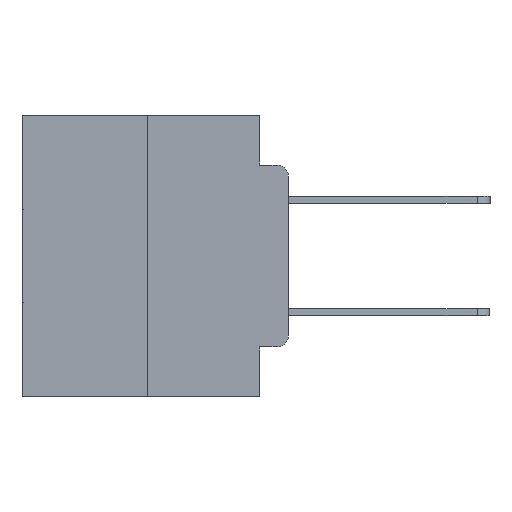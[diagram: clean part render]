
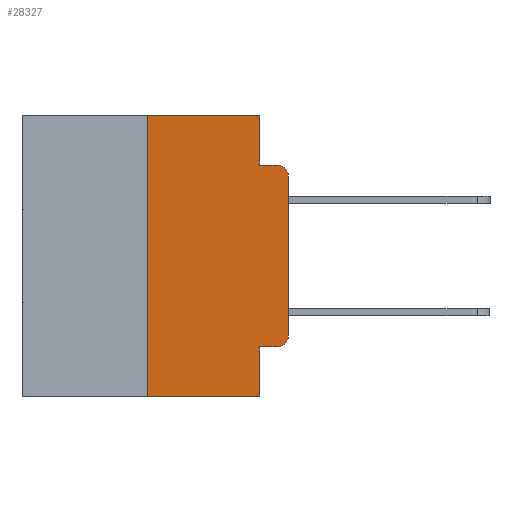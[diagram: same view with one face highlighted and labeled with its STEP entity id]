
A CAD part, left-side view. The second image highlights one B-rep face of the part: STEP entity #28327.
In plain terms, the highlighted planar face has unit normal (-1, 0, 0).
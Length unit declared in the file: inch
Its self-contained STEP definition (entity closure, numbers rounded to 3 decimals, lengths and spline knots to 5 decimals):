
#244 = CARTESIAN_POINT ( 'NONE',  ( 0., 0., -0.3915 ) ) ;
#656 = CARTESIAN_POINT ( 'NONE',  ( 0., 0.02, -0.1085 ) ) ;
#771 = DIRECTION ( 'NONE',  ( 0., 0., -1. ) ) ;
#1029 = ORIENTED_EDGE ( 'NONE', *, *, #26617, .F. ) ;
#1486 = CARTESIAN_POINT ( 'NONE',  ( 0., 0.25, 0. ) ) ;
#2059 = EDGE_CURVE ( 'NONE', #5785, #24473, #16417, .T. ) ;
#2586 = VERTEX_POINT ( 'NONE', #22466 ) ;
#2895 = CARTESIAN_POINT ( 'NONE',  ( 0., 0., 0. ) ) ;
#3025 = DIRECTION ( 'NONE',  ( 0., 0., -1. ) ) ;
#3027 = AXIS2_PLACEMENT_3D ( 'NONE', #18793, #18895, #5268 ) ;
#3279 = LINE ( 'NONE', #20834, #20783 ) ;
#3601 = VECTOR ( 'NONE', #771, 39.37008 ) ;
#3701 = CARTESIAN_POINT ( 'NONE',  ( 0., 0.02, -0.3915 ) ) ;
#3766 = LINE ( 'NONE', #16473, #15129 ) ;
#4317 = ORIENTED_EDGE ( 'NONE', *, *, #14441, .T. ) ;
#4804 = AXIS2_PLACEMENT_3D ( 'NONE', #656, #16676, #3025 ) ;
#5252 = DIRECTION ( 'NONE',  ( 0., -1., 0. ) ) ;
#5268 = DIRECTION ( 'NONE',  ( 0., 0., -1. ) ) ;
#5785 = VERTEX_POINT ( 'NONE', #28866 ) ;
#5810 = EDGE_LOOP ( 'NONE', ( #4317, #24004, #11480, #17840, #15767, #1029, #19303, #20393, #8933, #7186 ) ) ;
#5826 = VECTOR ( 'NONE', #21119, 39.37008 ) ;
#5998 = DIRECTION ( 'NONE',  ( 0., 0., -1. ) ) ;
#6046 = VERTEX_POINT ( 'NONE', #9480 ) ;
#7186 = ORIENTED_EDGE ( 'NONE', *, *, #18304, .T. ) ;
#7313 = CARTESIAN_POINT ( 'NONE',  ( 0., 0.051, -0.0885 ) ) ;
#7432 = VERTEX_POINT ( 'NONE', #16982 ) ;
#8602 = CIRCLE ( 'NONE', #4804, 0.02 ) ;
#8619 = CIRCLE ( 'NONE', #14096, 0.02 ) ;
#8933 = ORIENTED_EDGE ( 'NONE', *, *, #21608, .T. ) ;
#9033 = CARTESIAN_POINT ( 'NONE',  ( 0., 0.051, 0. ) ) ;
#9480 = CARTESIAN_POINT ( 'NONE',  ( 0., 0.051, -0.5 ) ) ;
#10533 = VECTOR ( 'NONE', #18191, 39.37008 ) ;
#10970 = VECTOR ( 'NONE', #14238, 39.37008 ) ;
#11480 = ORIENTED_EDGE ( 'NONE', *, *, #17508, .F. ) ;
#11672 = LINE ( 'NONE', #2895, #10970 ) ;
#11962 = EDGE_CURVE ( 'NONE', #13282, #23412, #8602, .T. ) ;
#11974 = CARTESIAN_POINT ( 'NONE',  ( 0., 0.473, -0.5 ) ) ;
#12280 = FACE_OUTER_BOUND ( 'NONE', #5810, .T. ) ;
#12442 = CARTESIAN_POINT ( 'NONE',  ( 0., 0.051, -0.0885 ) ) ;
#12578 = CARTESIAN_POINT ( 'NONE',  ( 0., 0.051, 0. ) ) ;
#13282 = VERTEX_POINT ( 'NONE', #19433 ) ;
#14096 = AXIS2_PLACEMENT_3D ( 'NONE', #3701, #19671, #5998 ) ;
#14238 = DIRECTION ( 'NONE',  ( 0., 0., 1. ) ) ;
#14441 = EDGE_CURVE ( 'NONE', #23753, #13282, #11672, .T. ) ;
#15129 = VECTOR ( 'NONE', #18777, 39.37008 ) ;
#15767 = ORIENTED_EDGE ( 'NONE', *, *, #16295, .F. ) ;
#16295 = EDGE_CURVE ( 'NONE', #25643, #5785, #3766, .T. ) ;
#16417 = LINE ( 'NONE', #12578, #3601 ) ;
#16473 = CARTESIAN_POINT ( 'NONE',  ( 0., 0.473, 0. ) ) ;
#16529 = LINE ( 'NONE', #1486, #22661 ) ;
#16585 = PLANE ( 'NONE',  #3027 ) ;
#16676 = DIRECTION ( 'NONE',  ( -1., 0., 0. ) ) ;
#16982 = CARTESIAN_POINT ( 'NONE',  ( 0., 0.051, -0.4115 ) ) ;
#17476 = DIRECTION ( 'NONE',  ( 0., 0., 1. ) ) ;
#17508 = EDGE_CURVE ( 'NONE', #24473, #23412, #25464, .T. ) ;
#17840 = ORIENTED_EDGE ( 'NONE', *, *, #2059, .F. ) ;
#18191 = DIRECTION ( 'NONE',  ( 0., 0., -1. ) ) ;
#18304 = EDGE_CURVE ( 'NONE', #2586, #23753, #8619, .T. ) ;
#18777 = DIRECTION ( 'NONE',  ( 0., -1., 0. ) ) ;
#18793 = CARTESIAN_POINT ( 'NONE',  ( 0., 0.473, 0. ) ) ;
#18895 = DIRECTION ( 'NONE',  ( 1., 0., 0. ) ) ;
#19303 = ORIENTED_EDGE ( 'NONE', *, *, #19400, .T. ) ;
#19400 = EDGE_CURVE ( 'NONE', #20803, #6046, #27834, .T. ) ;
#19433 = CARTESIAN_POINT ( 'NONE',  ( 0., 0., -0.1085 ) ) ;
#19671 = DIRECTION ( 'NONE',  ( -1., 0., 0. ) ) ;
#20393 = ORIENTED_EDGE ( 'NONE', *, *, #28137, .F. ) ;
#20783 = VECTOR ( 'NONE', #27581, 39.37008 ) ;
#20803 = VERTEX_POINT ( 'NONE', #24458 ) ;
#20834 = CARTESIAN_POINT ( 'NONE',  ( 0., 0.051, -0.4115 ) ) ;
#21119 = DIRECTION ( 'NONE',  ( 0., -1., 0. ) ) ;
#21608 = EDGE_CURVE ( 'NONE', #7432, #2586, #3279, .T. ) ;
#21805 = VECTOR ( 'NONE', #5252, 39.37008 ) ;
#22466 = CARTESIAN_POINT ( 'NONE',  ( 0., 0.02, -0.4115 ) ) ;
#22661 = VECTOR ( 'NONE', #17476, 39.37008 ) ;
#23412 = VERTEX_POINT ( 'NONE', #26427 ) ;
#23753 = VERTEX_POINT ( 'NONE', #244 ) ;
#24004 = ORIENTED_EDGE ( 'NONE', *, *, #11962, .T. ) ;
#24458 = CARTESIAN_POINT ( 'NONE',  ( 0., 0.25, -0.5 ) ) ;
#24473 = VERTEX_POINT ( 'NONE', #12442 ) ;
#25464 = LINE ( 'NONE', #7313, #5826 ) ;
#25643 = VERTEX_POINT ( 'NONE', #27890 ) ;
#26427 = CARTESIAN_POINT ( 'NONE',  ( 0., 0.02, -0.0885 ) ) ;
#26617 = EDGE_CURVE ( 'NONE', #20803, #25643, #16529, .T. ) ;
#27581 = DIRECTION ( 'NONE',  ( 0., -1., 0. ) ) ;
#27834 = LINE ( 'NONE', #11974, #21805 ) ;
#27890 = CARTESIAN_POINT ( 'NONE',  ( 0., 0.25, 0. ) ) ;
#28137 = EDGE_CURVE ( 'NONE', #7432, #6046, #29461, .T. ) ;
#28327 = ADVANCED_FACE ( 'NONE', ( #12280 ), #16585, .F. ) ;
#28866 = CARTESIAN_POINT ( 'NONE',  ( 0., 0.051, 0. ) ) ;
#29461 = LINE ( 'NONE', #9033, #10533 ) ;
